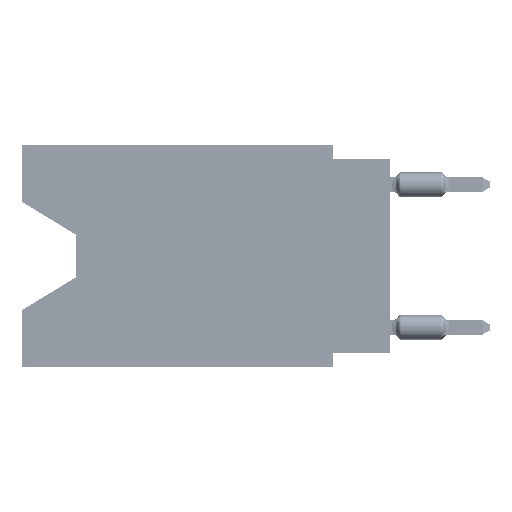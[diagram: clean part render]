
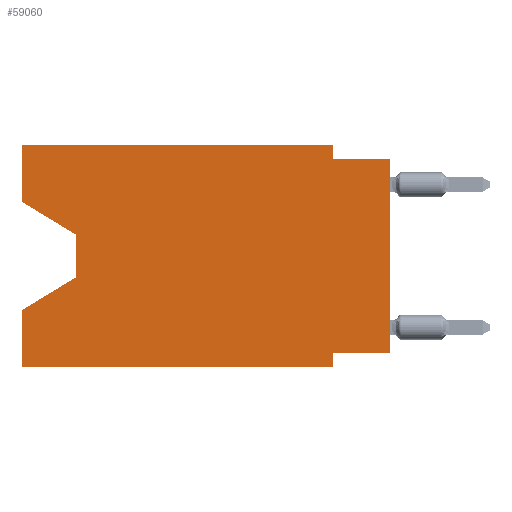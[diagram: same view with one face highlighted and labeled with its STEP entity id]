
A CAD part, left-side view. The second image highlights one B-rep face of the part: STEP entity #59060.
In plain terms, the highlighted planar face has unit normal (-1, 0, 0).
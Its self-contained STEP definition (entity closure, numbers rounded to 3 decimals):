
#741 = VERTEX_POINT ( 'NONE', #20261 ) ;
#2409 = LINE ( 'NONE', #29752, #31180 ) ;
#4786 = CARTESIAN_POINT ( 'NONE',  ( 0., 2.54, 0. ) ) ;
#4868 = CARTESIAN_POINT ( 'NONE',  ( 0., 0., -0.635 ) ) ;
#5183 = DIRECTION ( 'NONE',  ( 0., 0., -1. ) ) ;
#6454 = CARTESIAN_POINT ( 'NONE',  ( 0., 16.383, -7.36 ) ) ;
#6588 = CARTESIAN_POINT ( 'NONE',  ( 0., 16.383, -9.906 ) ) ;
#6597 = CARTESIAN_POINT ( 'NONE',  ( 0., 2.54, -9.906 ) ) ;
#6703 = LINE ( 'NONE', #48866, #64839 ) ;
#6746 = LINE ( 'NONE', #7639, #79426 ) ;
#7121 = CARTESIAN_POINT ( 'NONE',  ( 0., 16.383, 0. ) ) ;
#7639 = CARTESIAN_POINT ( 'NONE',  ( 0., 16.383, -9.906 ) ) ;
#9569 = EDGE_CURVE ( 'NONE', #50415, #30185, #55984, .T. ) ;
#11830 = DIRECTION ( 'NONE',  ( 0., 0.855, -0.519 ) ) ;
#11901 = VERTEX_POINT ( 'NONE', #71411 ) ;
#12403 = VERTEX_POINT ( 'NONE', #80145 ) ;
#14554 = EDGE_CURVE ( 'NONE', #27087, #741, #79353, .T. ) ;
#15826 = VECTOR ( 'NONE', #62673, 1000. ) ;
#16461 = LINE ( 'NONE', #57284, #56997 ) ;
#17126 = VERTEX_POINT ( 'NONE', #75390 ) ;
#17714 = VECTOR ( 'NONE', #31785, 1000. ) ;
#18243 = DIRECTION ( 'NONE',  ( 0., 0., -1. ) ) ;
#19433 = LINE ( 'NONE', #46367, #60175 ) ;
#20261 = CARTESIAN_POINT ( 'NONE',  ( 0., 2.54, -9.271 ) ) ;
#21048 = DIRECTION ( 'NONE',  ( 0., -0.855, -0.519 ) ) ;
#22298 = DIRECTION ( 'NONE',  ( 0., 0., 1. ) ) ;
#24180 = CARTESIAN_POINT ( 'NONE',  ( 0., 16.383, -2.546 ) ) ;
#27087 = VERTEX_POINT ( 'NONE', #43702 ) ;
#27929 = EDGE_LOOP ( 'NONE', ( #52984, #45437, #56904, #31420, #36238, #47464, #70333, #53260, #29619, #43620, #68234, #42542 ) ) ;
#28424 = VECTOR ( 'NONE', #39416, 1000. ) ;
#29619 = ORIENTED_EDGE ( 'NONE', *, *, #53058, .F. ) ;
#29752 = CARTESIAN_POINT ( 'NONE',  ( 0., 16.383, 0. ) ) ;
#30185 = VERTEX_POINT ( 'NONE', #68678 ) ;
#30305 = EDGE_CURVE ( 'NONE', #68992, #50415, #46586, .T. ) ;
#31180 = VECTOR ( 'NONE', #57134, 1000. ) ;
#31420 = ORIENTED_EDGE ( 'NONE', *, *, #49961, .F. ) ;
#31785 = DIRECTION ( 'NONE',  ( 0., -1., 0. ) ) ;
#32019 = EDGE_CURVE ( 'NONE', #17126, #54108, #19433, .T. ) ;
#32975 = LINE ( 'NONE', #74669, #39099 ) ;
#33957 = DIRECTION ( 'NONE',  ( 0., 0., -1. ) ) ;
#36035 = DIRECTION ( 'NONE',  ( 1., 0., 0. ) ) ;
#36238 = ORIENTED_EDGE ( 'NONE', *, *, #80284, .T. ) ;
#36785 = AXIS2_PLACEMENT_3D ( 'NONE', #43204, #36035, #63422 ) ;
#39099 = VECTOR ( 'NONE', #5183, 1000. ) ;
#39416 = DIRECTION ( 'NONE',  ( 0., 0., 1. ) ) ;
#40116 = VERTEX_POINT ( 'NONE', #4868 ) ;
#42542 = ORIENTED_EDGE ( 'NONE', *, *, #30305, .F. ) ;
#43204 = CARTESIAN_POINT ( 'NONE',  ( 0., 16.383, 0. ) ) ;
#43620 = ORIENTED_EDGE ( 'NONE', *, *, #48561, .F. ) ;
#43702 = CARTESIAN_POINT ( 'NONE',  ( 0., 0., -9.271 ) ) ;
#45437 = ORIENTED_EDGE ( 'NONE', *, *, #52360, .T. ) ;
#46367 = CARTESIAN_POINT ( 'NONE',  ( 0., 13.97, -5.893 ) ) ;
#46586 = LINE ( 'NONE', #60049, #28424 ) ;
#47464 = ORIENTED_EDGE ( 'NONE', *, *, #52036, .F. ) ;
#48373 = EDGE_CURVE ( 'NONE', #27087, #40116, #16461, .T. ) ;
#48561 = EDGE_CURVE ( 'NONE', #30185, #11901, #60391, .T. ) ;
#48866 = CARTESIAN_POINT ( 'NONE',  ( 0., 16.383, -2.546 ) ) ;
#49255 = CARTESIAN_POINT ( 'NONE',  ( 0., 16.383, 0. ) ) ;
#49961 = EDGE_CURVE ( 'NONE', #75624, #54108, #2409, .T. ) ;
#50415 = VERTEX_POINT ( 'NONE', #7121 ) ;
#52036 = EDGE_CURVE ( 'NONE', #741, #12403, #68069, .T. ) ;
#52360 = EDGE_CURVE ( 'NONE', #62299, #17126, #32975, .T. ) ;
#52713 = CARTESIAN_POINT ( 'NONE',  ( 0., 13.97, -4.013 ) ) ;
#52984 = ORIENTED_EDGE ( 'NONE', *, *, #76464, .T. ) ;
#53058 = EDGE_CURVE ( 'NONE', #11901, #40116, #72173, .T. ) ;
#53260 = ORIENTED_EDGE ( 'NONE', *, *, #48373, .T. ) ;
#54108 = VERTEX_POINT ( 'NONE', #6454 ) ;
#54751 = DIRECTION ( 'NONE',  ( 0., -1., 0. ) ) ;
#55984 = LINE ( 'NONE', #49255, #77238 ) ;
#56904 = ORIENTED_EDGE ( 'NONE', *, *, #32019, .T. ) ;
#56997 = VECTOR ( 'NONE', #22298, 1000. ) ;
#57134 = DIRECTION ( 'NONE',  ( 0., 0., 1. ) ) ;
#57284 = CARTESIAN_POINT ( 'NONE',  ( 0., 0., 0. ) ) ;
#59060 = ADVANCED_FACE ( 'NONE', ( #84488 ), #76878, .F. ) ;
#60049 = CARTESIAN_POINT ( 'NONE',  ( 0., 16.383, 0. ) ) ;
#60175 = VECTOR ( 'NONE', #11830, 1000. ) ;
#60391 = LINE ( 'NONE', #4786, #87115 ) ;
#62282 = DIRECTION ( 'NONE',  ( 0., -1., 0. ) ) ;
#62299 = VERTEX_POINT ( 'NONE', #52713 ) ;
#62673 = DIRECTION ( 'NONE',  ( 0., 1., 0. ) ) ;
#63422 = DIRECTION ( 'NONE',  ( 0., 0., -1. ) ) ;
#64839 = VECTOR ( 'NONE', #21048, 1000. ) ;
#64915 = VECTOR ( 'NONE', #33957, 1000. ) ;
#65004 = CARTESIAN_POINT ( 'NONE',  ( 0., 0., -0.635 ) ) ;
#68069 = LINE ( 'NONE', #6597, #64915 ) ;
#68234 = ORIENTED_EDGE ( 'NONE', *, *, #9569, .F. ) ;
#68678 = CARTESIAN_POINT ( 'NONE',  ( 0., 2.54, 0. ) ) ;
#68992 = VERTEX_POINT ( 'NONE', #24180 ) ;
#70333 = ORIENTED_EDGE ( 'NONE', *, *, #14554, .F. ) ;
#71411 = CARTESIAN_POINT ( 'NONE',  ( 0., 2.54, -0.635 ) ) ;
#72173 = LINE ( 'NONE', #65004, #17714 ) ;
#74669 = CARTESIAN_POINT ( 'NONE',  ( 0., 13.97, -4.013 ) ) ;
#75390 = CARTESIAN_POINT ( 'NONE',  ( 0., 13.97, -5.893 ) ) ;
#75624 = VERTEX_POINT ( 'NONE', #6588 ) ;
#76464 = EDGE_CURVE ( 'NONE', #68992, #62299, #6703, .T. ) ;
#76878 = PLANE ( 'NONE',  #36785 ) ;
#77238 = VECTOR ( 'NONE', #62282, 1000. ) ;
#79353 = LINE ( 'NONE', #79789, #15826 ) ;
#79426 = VECTOR ( 'NONE', #54751, 1000. ) ;
#79789 = CARTESIAN_POINT ( 'NONE',  ( 0., 0., -9.271 ) ) ;
#80145 = CARTESIAN_POINT ( 'NONE',  ( 0., 2.54, -9.906 ) ) ;
#80284 = EDGE_CURVE ( 'NONE', #75624, #12403, #6746, .T. ) ;
#84488 = FACE_OUTER_BOUND ( 'NONE', #27929, .T. ) ;
#87115 = VECTOR ( 'NONE', #18243, 1000. ) ;
